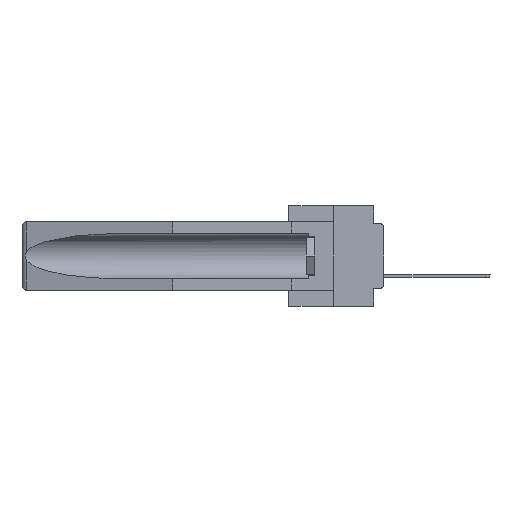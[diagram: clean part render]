
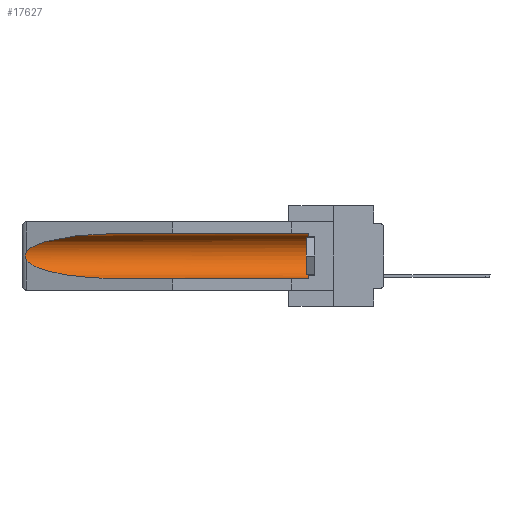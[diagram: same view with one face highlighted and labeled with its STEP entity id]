
A CAD part, left-side view. The second image highlights one B-rep face of the part: STEP entity #17627.
In plain terms, the highlighted cylindrical face has radius 2.857 mm (diameter 5.715 mm), a partial arc.
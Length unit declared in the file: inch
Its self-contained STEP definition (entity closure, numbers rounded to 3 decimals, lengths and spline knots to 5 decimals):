
#238 = VERTEX_POINT ( 'NONE', #1811 ) ;
#615 = B_SPLINE_CURVE_WITH_KNOTS ( 'NONE', 3,
 ( #1621, #3833, #6235, #25247, #11310, #8443, #1298, #30361, #13602, #13180 ),
 .UNSPECIFIED., .F., .F.,
 ( 4, 2, 2, 2, 4 ),
 ( 0., 0.00029, 0.00058, 0.00087, 0.00117 ),
 .UNSPECIFIED. ) ;
#701 = CARTESIAN_POINT ( 'NONE',  ( 0.155, 1.07973, -0.284 ) ) ;
#1266 = CARTESIAN_POINT ( 'NONE',  ( 0.155, -0.30754, -0.1715 ) ) ;
#1298 = CARTESIAN_POINT ( 'NONE',  ( 0.2673, 1.53269, -0.17917 ) ) ;
#1621 = CARTESIAN_POINT ( 'NONE',  ( 0.26537, 1.52718, -0.14972 ) ) ;
#1811 = CARTESIAN_POINT ( 'NONE',  ( 0.155, 0.126, -0.059 ) ) ;
#2525 = VECTOR ( 'NONE', #25037, 39.37008 ) ;
#3833 = CARTESIAN_POINT ( 'NONE',  ( 0.26597, 1.52961, -0.15275 ) ) ;
#4095 = VERTEX_POINT ( 'NONE', #5471 ) ;
#4296 =( BOUNDED_CURVE ( )  B_SPLINE_CURVE ( 3, ( #11595, #21229, #6840, #16125 ),
 .UNSPECIFIED., .F., .F. ) 
 B_SPLINE_CURVE_WITH_KNOTS ( ( 4, 4 ),
 ( 0.1948, 1.5708 ),
 .UNSPECIFIED. ) 
 CURVE ( )  GEOMETRIC_REPRESENTATION_ITEM ( )  RATIONAL_B_SPLINE_CURVE ( ( 1., 0.848, 0.848, 1. ) ) 
 REPRESENTATION_ITEM ( '' )  );
#4390 = DIRECTION ( 'NONE',  ( 0., 1., 0. ) ) ;
#5079 = DIRECTION ( 'NONE',  ( 0., 0., 1. ) ) ;
#5115 = CYLINDRICAL_SURFACE ( 'NONE', #15620, 0.1125 ) ;
#5471 = CARTESIAN_POINT ( 'NONE',  ( 0.26537, 1.52718, -0.19328 ) ) ;
#6235 = CARTESIAN_POINT ( 'NONE',  ( 0.26654, 1.53092, -0.15636 ) ) ;
#6840 = CARTESIAN_POINT ( 'NONE',  ( 0.21114, 1.30732, -0.284 ) ) ;
#7519 = EDGE_CURVE ( 'NONE', #8824, #238, #27671, .T. ) ;
#7699 = EDGE_CURVE ( 'NONE', #8824, #18648, #16094, .T. ) ;
#8443 = CARTESIAN_POINT ( 'NONE',  ( 0.2675, 1.53308, -0.17534 ) ) ;
#8824 = VERTEX_POINT ( 'NONE', #29719 ) ;
#8880 = FACE_OUTER_BOUND ( 'NONE', #21993, .T. ) ;
#9787 = ORIENTED_EDGE ( 'NONE', *, *, #16926, .T. ) ;
#9948 = CARTESIAN_POINT ( 'NONE',  ( 0.25451, 1.48313, -0.09465 ) ) ;
#11065 = DIRECTION ( 'NONE',  ( 0., 0., 1. ) ) ;
#11310 = CARTESIAN_POINT ( 'NONE',  ( 0.2675, 1.53308, -0.16763 ) ) ;
#11408 = VERTEX_POINT ( 'NONE', #20584 ) ;
#11595 = CARTESIAN_POINT ( 'NONE',  ( 0.26537, 1.52718, -0.19328 ) ) ;
#13180 = CARTESIAN_POINT ( 'NONE',  ( 0.26537, 1.52718, -0.19328 ) ) ;
#13355 = DIRECTION ( 'NONE',  ( 0., 1., 0. ) ) ;
#13602 = CARTESIAN_POINT ( 'NONE',  ( 0.26597, 1.5296, -0.19026 ) ) ;
#13942 = CARTESIAN_POINT ( 'NONE',  ( 0.155, 1.07973, -0.059 ) ) ;
#15334 = ORIENTED_EDGE ( 'NONE', *, *, #7519, .T. ) ;
#15620 = AXIS2_PLACEMENT_3D ( 'NONE', #1266, #13355, #11065 ) ;
#16094 = LINE ( 'NONE', #17825, #2525 ) ;
#16125 = CARTESIAN_POINT ( 'NONE',  ( 0.155, 1.07973, -0.284 ) ) ;
#16466 = VECTOR ( 'NONE', #4390, 39.37008 ) ;
#16577 = ORIENTED_EDGE ( 'NONE', *, *, #29984, .T. ) ;
#16830 = ORIENTED_EDGE ( 'NONE', *, *, #7699, .F. ) ;
#16926 = EDGE_CURVE ( 'NONE', #28703, #4095, #615, .T. ) ;
#17170 = CARTESIAN_POINT ( 'NONE',  ( 0.155, 0.126, -0.1715 ) ) ;
#17627 = ADVANCED_FACE ( 'NONE', ( #8880 ), #5115, .F. ) ;
#17825 = CARTESIAN_POINT ( 'NONE',  ( 0.155, -0.30754, -0.284 ) ) ;
#18648 = VERTEX_POINT ( 'NONE', #701 ) ;
#19112 = CARTESIAN_POINT ( 'NONE',  ( 0.155, -0.30754, -0.059 ) ) ;
#20584 = CARTESIAN_POINT ( 'NONE',  ( 0.155, 1.07973, -0.059 ) ) ;
#21229 = CARTESIAN_POINT ( 'NONE',  ( 0.25451, 1.48313, -0.24835 ) ) ;
#21854 = EDGE_CURVE ( 'NONE', #11408, #28703, #30253, .T. ) ;
#21993 = EDGE_LOOP ( 'NONE', ( #26748, #9787, #29084, #16830, #15334, #16577 ) ) ;
#22628 = AXIS2_PLACEMENT_3D ( 'NONE', #17170, #29098, #5079 ) ;
#23367 = EDGE_CURVE ( 'NONE', #4095, #18648, #4296, .T. ) ;
#23529 = CARTESIAN_POINT ( 'NONE',  ( 0.26537, 1.52718, -0.14972 ) ) ;
#23577 = LINE ( 'NONE', #19112, #16466 ) ;
#23588 = CARTESIAN_POINT ( 'NONE',  ( 0.21114, 1.30732, -0.059 ) ) ;
#25037 = DIRECTION ( 'NONE',  ( 0., 1., 0. ) ) ;
#25247 = CARTESIAN_POINT ( 'NONE',  ( 0.2673, 1.5327, -0.16383 ) ) ;
#26420 = CARTESIAN_POINT ( 'NONE',  ( 0.26537, 1.52718, -0.14972 ) ) ;
#26748 = ORIENTED_EDGE ( 'NONE', *, *, #21854, .T. ) ;
#27671 = CIRCLE ( 'NONE', #22628, 0.1125 ) ;
#28703 = VERTEX_POINT ( 'NONE', #23529 ) ;
#29084 = ORIENTED_EDGE ( 'NONE', *, *, #23367, .T. ) ;
#29098 = DIRECTION ( 'NONE',  ( 0., -1., 0. ) ) ;
#29719 = CARTESIAN_POINT ( 'NONE',  ( 0.155, 0.126, -0.284 ) ) ;
#29984 = EDGE_CURVE ( 'NONE', #238, #11408, #23577, .T. ) ;
#30253 =( BOUNDED_CURVE ( )  B_SPLINE_CURVE ( 3, ( #13942, #23588, #9948, #26420 ),
 .UNSPECIFIED., .F., .F. ) 
 B_SPLINE_CURVE_WITH_KNOTS ( ( 4, 4 ),
 ( 4.71239, 6.08839 ),
 .UNSPECIFIED. ) 
 CURVE ( )  GEOMETRIC_REPRESENTATION_ITEM ( )  RATIONAL_B_SPLINE_CURVE ( ( 1., 0.848, 0.848, 1. ) ) 
 REPRESENTATION_ITEM ( '' )  );
#30361 = CARTESIAN_POINT ( 'NONE',  ( 0.26655, 1.53094, -0.18657 ) ) ;
